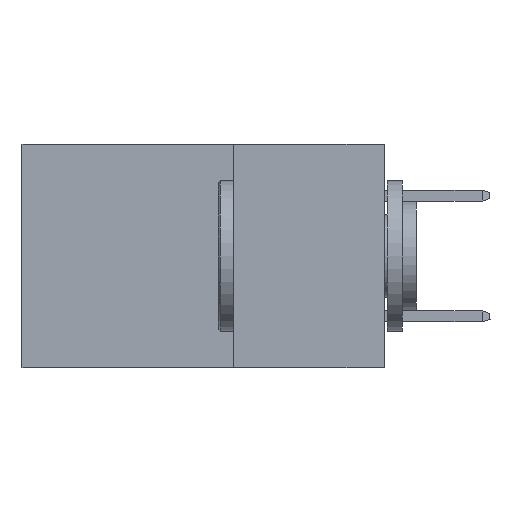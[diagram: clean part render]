
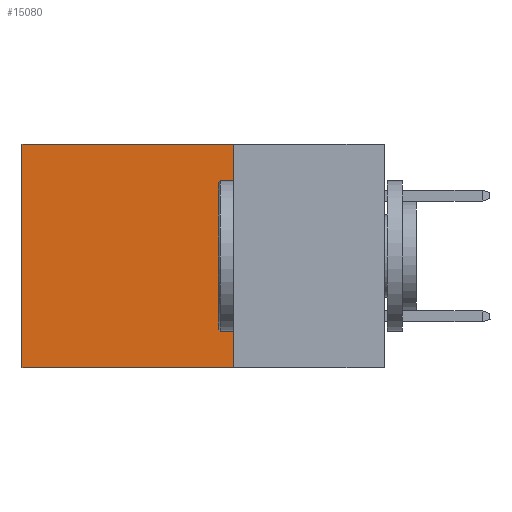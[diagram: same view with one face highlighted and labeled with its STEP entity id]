
A CAD part, left-side view. The second image highlights one B-rep face of the part: STEP entity #15080.
In plain terms, the highlighted planar face has unit normal (-1, 0, 0).
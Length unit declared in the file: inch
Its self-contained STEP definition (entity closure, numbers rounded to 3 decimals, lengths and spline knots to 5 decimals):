
#218 = VERTEX_POINT ( 'NONE', #22003 ) ;
#1928 = DIRECTION ( 'NONE',  ( 0., 0., -1. ) ) ;
#2790 = EDGE_CURVE ( 'NONE', #11372, #14058, #19298, .T. ) ;
#3014 = CARTESIAN_POINT ( 'NONE',  ( 0.2615, 0.25, -0.37 ) ) ;
#3080 = EDGE_CURVE ( 'NONE', #218, #14058, #8177, .T. ) ;
#3261 = CARTESIAN_POINT ( 'NONE',  ( 0.2615, 0.25, 0. ) ) ;
#3424 = ORIENTED_EDGE ( 'NONE', *, *, #15369, .T. ) ;
#4460 = CARTESIAN_POINT ( 'NONE',  ( 0.2615, 0.25, 0. ) ) ;
#5835 = AXIS2_PLACEMENT_3D ( 'NONE', #10629, #12319, #1928 ) ;
#6037 = EDGE_LOOP ( 'NONE', ( #13074, #20171, #8863, #3424 ) ) ;
#7790 = VECTOR ( 'NONE', #14784, 39.37008 ) ;
#8177 = LINE ( 'NONE', #12614, #17734 ) ;
#8863 = ORIENTED_EDGE ( 'NONE', *, *, #13546, .F. ) ;
#8880 = PLANE ( 'NONE',  #5835 ) ;
#10026 = DIRECTION ( 'NONE',  ( 0., 1., 0. ) ) ;
#10629 = CARTESIAN_POINT ( 'NONE',  ( 0.2615, 0.25, -0.37 ) ) ;
#10835 = VERTEX_POINT ( 'NONE', #3261 ) ;
#10871 = CARTESIAN_POINT ( 'NONE',  ( 0.2615, 0.25, -0.37 ) ) ;
#11372 = VERTEX_POINT ( 'NONE', #3014 ) ;
#12319 = DIRECTION ( 'NONE',  ( 1., 0., 0. ) ) ;
#12326 = LINE ( 'NONE', #4460, #7790 ) ;
#12519 = DIRECTION ( 'NONE',  ( 0., 0., -1. ) ) ;
#12614 = CARTESIAN_POINT ( 'NONE',  ( 0.2615, 0.6, -0.37 ) ) ;
#13074 = ORIENTED_EDGE ( 'NONE', *, *, #3080, .T. ) ;
#13546 = EDGE_CURVE ( 'NONE', #10835, #11372, #21305, .T. ) ;
#14058 = VERTEX_POINT ( 'NONE', #14808 ) ;
#14784 = DIRECTION ( 'NONE',  ( 0., 1., 0. ) ) ;
#14808 = CARTESIAN_POINT ( 'NONE',  ( 0.2615, 0.6, -0.37 ) ) ;
#15080 = ADVANCED_FACE ( 'NONE', ( #18146 ), #8880, .F. ) ;
#15369 = EDGE_CURVE ( 'NONE', #10835, #218, #12326, .T. ) ;
#16399 = VECTOR ( 'NONE', #20268, 39.37008 ) ;
#17734 = VECTOR ( 'NONE', #12519, 39.37008 ) ;
#18146 = FACE_OUTER_BOUND ( 'NONE', #6037, .T. ) ;
#18774 = VECTOR ( 'NONE', #10026, 39.37008 ) ;
#19298 = LINE ( 'NONE', #10871, #18774 ) ;
#20171 = ORIENTED_EDGE ( 'NONE', *, *, #2790, .F. ) ;
#20268 = DIRECTION ( 'NONE',  ( 0., 0., -1. ) ) ;
#21305 = LINE ( 'NONE', #21843, #16399 ) ;
#21843 = CARTESIAN_POINT ( 'NONE',  ( 0.2615, 0.25, -0.37 ) ) ;
#22003 = CARTESIAN_POINT ( 'NONE',  ( 0.2615, 0.6, 0. ) ) ;
